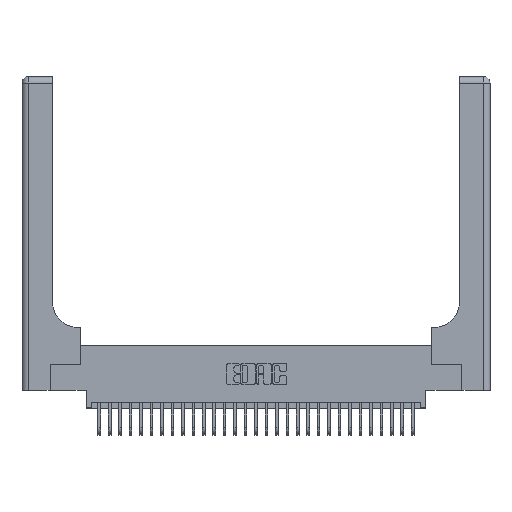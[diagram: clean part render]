
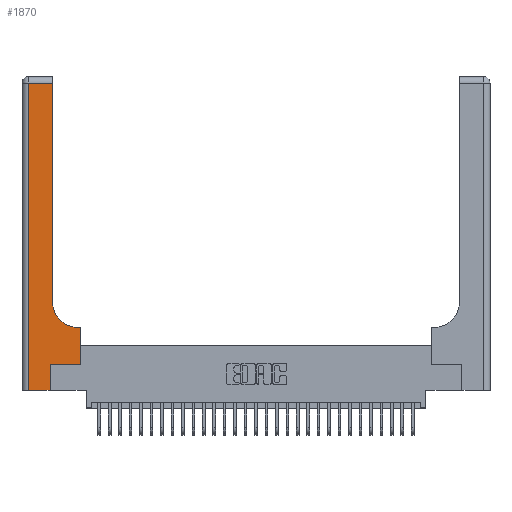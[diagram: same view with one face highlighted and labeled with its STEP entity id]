
A CAD part, top view. The second image highlights one B-rep face of the part: STEP entity #1870.
In plain terms, the highlighted planar face has unit normal (0, 0, 1).
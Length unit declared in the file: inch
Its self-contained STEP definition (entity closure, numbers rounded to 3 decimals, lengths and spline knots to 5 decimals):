
#144 = DIRECTION ( 'NONE',  ( 1., 0., 0. ) ) ;
#233 = VECTOR ( 'NONE', #144, 39.37008 ) ;
#368 = DIRECTION ( 'NONE',  ( 0., 1., 0. ) ) ;
#521 = VECTOR ( 'NONE', #8176, 39.37008 ) ;
#589 = VERTEX_POINT ( 'NONE', #9736 ) ;
#1870 = ADVANCED_FACE ( 'NONE', ( #5853 ), #24810, .F. ) ;
#1968 = EDGE_CURVE ( 'NONE', #12268, #15574, #10679, .T. ) ;
#2919 = VERTEX_POINT ( 'NONE', #25706 ) ;
#3673 = CARTESIAN_POINT ( 'NONE',  ( 0.2915, 2.94, 0.37 ) ) ;
#4461 = CARTESIAN_POINT ( 'NONE',  ( 0.5415, 0.85, 0.37 ) ) ;
#4469 = ORIENTED_EDGE ( 'NONE', *, *, #14244, .T. ) ;
#5184 = CIRCLE ( 'NONE', #32743, 0.25 ) ;
#5293 = CARTESIAN_POINT ( 'NONE',  ( 0.5415, 0.6, 0.37 ) ) ;
#5659 = VERTEX_POINT ( 'NONE', #11283 ) ;
#5853 = FACE_OUTER_BOUND ( 'NONE', #32236, .T. ) ;
#5942 = DIRECTION ( 'NONE',  ( -1., 0., 0. ) ) ;
#6186 = VECTOR ( 'NONE', #5942, 39.37008 ) ;
#6562 = LINE ( 'NONE', #23352, #521 ) ;
#6745 = CARTESIAN_POINT ( 'NONE',  ( 0.269, 0.25, 0.37 ) ) ;
#6993 = AXIS2_PLACEMENT_3D ( 'NONE', #9666, #27307, #12221 ) ;
#7066 = DIRECTION ( 'NONE',  ( 1., 0., 0. ) ) ;
#7460 = CARTESIAN_POINT ( 'NONE',  ( 0.2915, 0.6, 0.37 ) ) ;
#8049 = CARTESIAN_POINT ( 'NONE',  ( 0.5585, 0.25, 0.37 ) ) ;
#8176 = DIRECTION ( 'NONE',  ( 0., -1., 0. ) ) ;
#8931 = ORIENTED_EDGE ( 'NONE', *, *, #13721, .T. ) ;
#9097 = ORIENTED_EDGE ( 'NONE', *, *, #1968, .T. ) ;
#9137 = LINE ( 'NONE', #7460, #29239 ) ;
#9462 = ORIENTED_EDGE ( 'NONE', *, *, #16527, .T. ) ;
#9666 = CARTESIAN_POINT ( 'NONE',  ( 0., 3., 0.37 ) ) ;
#9684 = VECTOR ( 'NONE', #30864, 39.37008 ) ;
#9736 = CARTESIAN_POINT ( 'NONE',  ( 0.06, 0., 0.37 ) ) ;
#10679 = LINE ( 'NONE', #30132, #24153 ) ;
#10776 = DIRECTION ( 'NONE',  ( 1., 0., 0. ) ) ;
#11283 = CARTESIAN_POINT ( 'NONE',  ( 0.5585, 0.6, 0.37 ) ) ;
#12221 = DIRECTION ( 'NONE',  ( -1., 0., 0. ) ) ;
#12268 = VERTEX_POINT ( 'NONE', #21679 ) ;
#12541 = DIRECTION ( 'NONE',  ( 0., 1., 0. ) ) ;
#12982 = LINE ( 'NONE', #26203, #6186 ) ;
#13307 = CARTESIAN_POINT ( 'NONE',  ( 0.269, 0., 0.37 ) ) ;
#13721 = EDGE_CURVE ( 'NONE', #589, #25632, #13893, .T. ) ;
#13893 = LINE ( 'NONE', #20617, #233 ) ;
#14244 = EDGE_CURVE ( 'NONE', #5659, #29822, #9137, .T. ) ;
#15132 = VECTOR ( 'NONE', #368, 39.37008 ) ;
#15574 = VERTEX_POINT ( 'NONE', #3673 ) ;
#15684 = LINE ( 'NONE', #13307, #9684 ) ;
#16527 = EDGE_CURVE ( 'NONE', #20267, #2919, #26049, .T. ) ;
#17237 = EDGE_CURVE ( 'NONE', #15574, #24768, #12982, .T. ) ;
#18727 = EDGE_CURVE ( 'NONE', #25632, #20267, #15684, .T. ) ;
#20267 = VERTEX_POINT ( 'NONE', #6745 ) ;
#20617 = CARTESIAN_POINT ( 'NONE',  ( 0., 0., 0.37 ) ) ;
#20969 = VECTOR ( 'NONE', #10776, 39.37008 ) ;
#21679 = CARTESIAN_POINT ( 'NONE',  ( 0.2915, 0.85, 0.37 ) ) ;
#21917 = ORIENTED_EDGE ( 'NONE', *, *, #30288, .T. ) ;
#22281 = DIRECTION ( 'NONE',  ( 0., 0., -1. ) ) ;
#22945 = EDGE_CURVE ( 'NONE', #24768, #589, #6562, .T. ) ;
#23352 = CARTESIAN_POINT ( 'NONE',  ( 0.06, 3., 0.37 ) ) ;
#23875 = CARTESIAN_POINT ( 'NONE',  ( 0.06, 2.94, 0.37 ) ) ;
#24153 = VECTOR ( 'NONE', #12541, 39.37008 ) ;
#24768 = VERTEX_POINT ( 'NONE', #23875 ) ;
#24810 = PLANE ( 'NONE',  #6993 ) ;
#25127 = CARTESIAN_POINT ( 'NONE',  ( 0.269, 0., 0.37 ) ) ;
#25163 = DIRECTION ( 'NONE',  ( -1., 0., 0. ) ) ;
#25632 = VERTEX_POINT ( 'NONE', #25127 ) ;
#25685 = ORIENTED_EDGE ( 'NONE', *, *, #18727, .T. ) ;
#25706 = CARTESIAN_POINT ( 'NONE',  ( 0.5585, 0.25, 0.37 ) ) ;
#26049 = LINE ( 'NONE', #28409, #20969 ) ;
#26203 = CARTESIAN_POINT ( 'NONE',  ( 0., 2.94, 0.37 ) ) ;
#27307 = DIRECTION ( 'NONE',  ( 0., 0., -1. ) ) ;
#28409 = CARTESIAN_POINT ( 'NONE',  ( 0.269, 0.25, 0.37 ) ) ;
#28467 = LINE ( 'NONE', #8049, #15132 ) ;
#29239 = VECTOR ( 'NONE', #25163, 39.37008 ) ;
#29822 = VERTEX_POINT ( 'NONE', #5293 ) ;
#30106 = ORIENTED_EDGE ( 'NONE', *, *, #22945, .T. ) ;
#30132 = CARTESIAN_POINT ( 'NONE',  ( 0.2915, 3., 0.37 ) ) ;
#30288 = EDGE_CURVE ( 'NONE', #29822, #12268, #5184, .T. ) ;
#30864 = DIRECTION ( 'NONE',  ( 0., 1., 0. ) ) ;
#31051 = EDGE_CURVE ( 'NONE', #2919, #5659, #28467, .T. ) ;
#31757 = ORIENTED_EDGE ( 'NONE', *, *, #17237, .T. ) ;
#32236 = EDGE_LOOP ( 'NONE', ( #9097, #31757, #30106, #8931, #25685, #9462, #32268, #4469, #21917 ) ) ;
#32268 = ORIENTED_EDGE ( 'NONE', *, *, #31051, .T. ) ;
#32743 = AXIS2_PLACEMENT_3D ( 'NONE', #4461, #22281, #7066 ) ;
